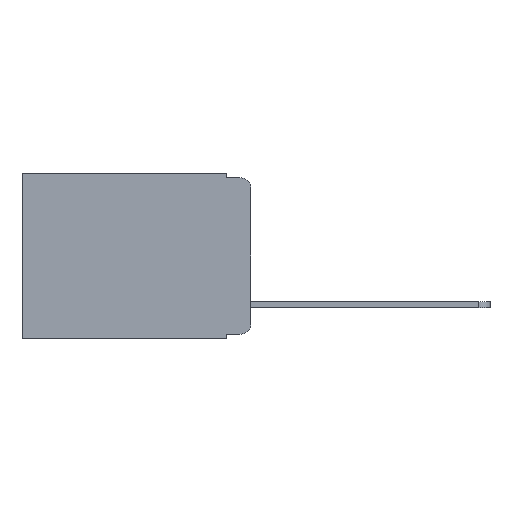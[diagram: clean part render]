
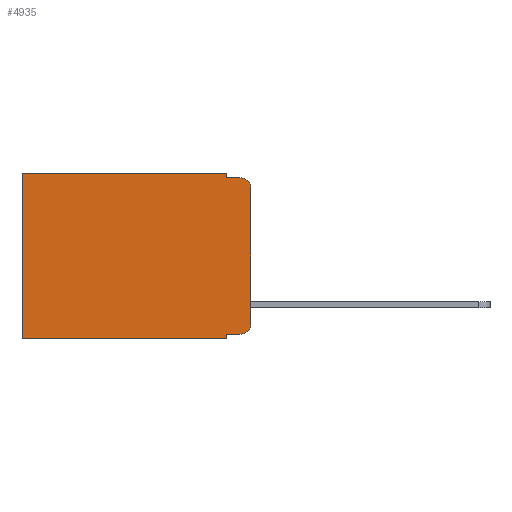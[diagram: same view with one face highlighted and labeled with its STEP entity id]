
A CAD part, left-side view. The second image highlights one B-rep face of the part: STEP entity #4935.
In plain terms, the highlighted planar face has unit normal (-1, 0, 0).
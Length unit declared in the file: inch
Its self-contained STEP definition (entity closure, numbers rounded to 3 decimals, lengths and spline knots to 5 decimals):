
#214 = LINE ( 'NONE', #12519, #8248 ) ;
#348 = ORIENTED_EDGE ( 'NONE', *, *, #10354, .F. ) ;
#513 = CIRCLE ( 'NONE', #12075, 0.02 ) ;
#734 = EDGE_LOOP ( 'NONE', ( #7172, #8774, #9420, #988, #1060, #5559, #348, #2787, #4647, #4472 ) ) ;
#957 = CARTESIAN_POINT ( 'NONE',  ( 0.298, 0.051, -0.343 ) ) ;
#988 = ORIENTED_EDGE ( 'NONE', *, *, #12541, .F. ) ;
#1060 = ORIENTED_EDGE ( 'NONE', *, *, #9520, .T. ) ;
#1316 = CARTESIAN_POINT ( 'NONE',  ( 0.298, 0.473, 0. ) ) ;
#1810 = PLANE ( 'NONE',  #10800 ) ;
#1953 = LINE ( 'NONE', #12665, #17043 ) ;
#2370 = FACE_OUTER_BOUND ( 'NONE', #734, .T. ) ;
#2534 = VERTEX_POINT ( 'NONE', #11144 ) ;
#2787 = ORIENTED_EDGE ( 'NONE', *, *, #11978, .F. ) ;
#3249 = EDGE_CURVE ( 'NONE', #10234, #10595, #1953, .T. ) ;
#4102 = CARTESIAN_POINT ( 'NONE',  ( 0.298, 0.473, -0.343 ) ) ;
#4264 = VERTEX_POINT ( 'NONE', #10282 ) ;
#4472 = ORIENTED_EDGE ( 'NONE', *, *, #14179, .T. ) ;
#4647 = ORIENTED_EDGE ( 'NONE', *, *, #12294, .T. ) ;
#4677 = DIRECTION ( 'NONE',  ( 0., 0., -1. ) ) ;
#4697 = CARTESIAN_POINT ( 'NONE',  ( 0.298, 0.02, -0.03 ) ) ;
#4764 = DIRECTION ( 'NONE',  ( -1., 0., 0. ) ) ;
#4935 = ADVANCED_FACE ( 'NONE', ( #2370 ), #1810, .F. ) ;
#5202 = LINE ( 'NONE', #18373, #16302 ) ;
#5559 = ORIENTED_EDGE ( 'NONE', *, *, #14885, .T. ) ;
#6053 = DIRECTION ( 'NONE',  ( 0., 0., -1. ) ) ;
#6326 = DIRECTION ( 'NONE',  ( 0., 0., -1. ) ) ;
#6378 = DIRECTION ( 'NONE',  ( 0., 0., -1. ) ) ;
#7079 = CARTESIAN_POINT ( 'NONE',  ( 0.298, 0.051, 0. ) ) ;
#7172 = ORIENTED_EDGE ( 'NONE', *, *, #3249, .F. ) ;
#7374 = DIRECTION ( 'NONE',  ( 0., -1., 0. ) ) ;
#7718 = VECTOR ( 'NONE', #6326, 39.37008 ) ;
#7901 = CARTESIAN_POINT ( 'NONE',  ( 0.298, 0., 0. ) ) ;
#7989 = CARTESIAN_POINT ( 'NONE',  ( 0.298, 0.02, -0.01 ) ) ;
#8248 = VECTOR ( 'NONE', #13940, 39.37008 ) ;
#8737 = DIRECTION ( 'NONE',  ( 0., 1., 0. ) ) ;
#8774 = ORIENTED_EDGE ( 'NONE', *, *, #14144, .T. ) ;
#8979 = EDGE_CURVE ( 'NONE', #2534, #11531, #13396, .T. ) ;
#9254 = VECTOR ( 'NONE', #8737, 39.37008 ) ;
#9420 = ORIENTED_EDGE ( 'NONE', *, *, #8979, .F. ) ;
#9426 = DIRECTION ( 'NONE',  ( 1., 0., 0. ) ) ;
#9520 = EDGE_CURVE ( 'NONE', #16247, #17940, #16561, .T. ) ;
#9552 = VERTEX_POINT ( 'NONE', #957 ) ;
#9955 = VERTEX_POINT ( 'NONE', #4102 ) ;
#10076 = VECTOR ( 'NONE', #6053, 39.37008 ) ;
#10234 = VERTEX_POINT ( 'NONE', #18569 ) ;
#10282 = CARTESIAN_POINT ( 'NONE',  ( 0.298, 0.02, -0.333 ) ) ;
#10354 = EDGE_CURVE ( 'NONE', #9552, #9955, #214, .T. ) ;
#10380 = LINE ( 'NONE', #18742, #13747 ) ;
#10595 = VERTEX_POINT ( 'NONE', #11892 ) ;
#10800 = AXIS2_PLACEMENT_3D ( 'NONE', #7901, #9426, #11178 ) ;
#11144 = CARTESIAN_POINT ( 'NONE',  ( 0.298, 0.051, -0.01 ) ) ;
#11178 = DIRECTION ( 'NONE',  ( 0., 0., -1. ) ) ;
#11531 = VERTEX_POINT ( 'NONE', #7989 ) ;
#11892 = CARTESIAN_POINT ( 'NONE',  ( 0.298, 0., -0.313 ) ) ;
#11978 = EDGE_CURVE ( 'NONE', #15455, #9552, #15362, .T. ) ;
#12075 = AXIS2_PLACEMENT_3D ( 'NONE', #4697, #15137, #6378 ) ;
#12088 = CARTESIAN_POINT ( 'NONE',  ( 0.298, 0.051, 0. ) ) ;
#12294 = EDGE_CURVE ( 'NONE', #15455, #4264, #5202, .T. ) ;
#12519 = CARTESIAN_POINT ( 'NONE',  ( 0.298, 0., -0.343 ) ) ;
#12541 = EDGE_CURVE ( 'NONE', #16247, #2534, #16841, .T. ) ;
#12665 = CARTESIAN_POINT ( 'NONE',  ( 0.298, 0., 0. ) ) ;
#12955 = VECTOR ( 'NONE', #18078, 39.37008 ) ;
#13014 = AXIS2_PLACEMENT_3D ( 'NONE', #13851, #4764, #15191 ) ;
#13396 = LINE ( 'NONE', #16827, #12955 ) ;
#13635 = DIRECTION ( 'NONE',  ( 0., 0., -1. ) ) ;
#13747 = VECTOR ( 'NONE', #4677, 39.37008 ) ;
#13851 = CARTESIAN_POINT ( 'NONE',  ( 0.298, 0.02, -0.313 ) ) ;
#13940 = DIRECTION ( 'NONE',  ( 0., 1., 0. ) ) ;
#14144 = EDGE_CURVE ( 'NONE', #10234, #11531, #513, .T. ) ;
#14179 = EDGE_CURVE ( 'NONE', #4264, #10595, #14411, .T. ) ;
#14411 = CIRCLE ( 'NONE', #13014, 0.02 ) ;
#14885 = EDGE_CURVE ( 'NONE', #17940, #9955, #10380, .T. ) ;
#15137 = DIRECTION ( 'NONE',  ( -1., 0., 0. ) ) ;
#15191 = DIRECTION ( 'NONE',  ( 0., 0., -1. ) ) ;
#15362 = LINE ( 'NONE', #16291, #7718 ) ;
#15455 = VERTEX_POINT ( 'NONE', #17889 ) ;
#16247 = VERTEX_POINT ( 'NONE', #7079 ) ;
#16291 = CARTESIAN_POINT ( 'NONE',  ( 0.298, 0.051, 0. ) ) ;
#16302 = VECTOR ( 'NONE', #7374, 39.37008 ) ;
#16561 = LINE ( 'NONE', #18202, #9254 ) ;
#16827 = CARTESIAN_POINT ( 'NONE',  ( 0.298, 0.051, -0.01 ) ) ;
#16841 = LINE ( 'NONE', #12088, #10076 ) ;
#17043 = VECTOR ( 'NONE', #13635, 39.37008 ) ;
#17889 = CARTESIAN_POINT ( 'NONE',  ( 0.298, 0.051, -0.333 ) ) ;
#17940 = VERTEX_POINT ( 'NONE', #1316 ) ;
#18078 = DIRECTION ( 'NONE',  ( 0., -1., 0. ) ) ;
#18202 = CARTESIAN_POINT ( 'NONE',  ( 0.298, 0., 0. ) ) ;
#18373 = CARTESIAN_POINT ( 'NONE',  ( 0.298, 0.051, -0.333 ) ) ;
#18569 = CARTESIAN_POINT ( 'NONE',  ( 0.298, 0., -0.03 ) ) ;
#18742 = CARTESIAN_POINT ( 'NONE',  ( 0.298, 0.473, 0. ) ) ;
